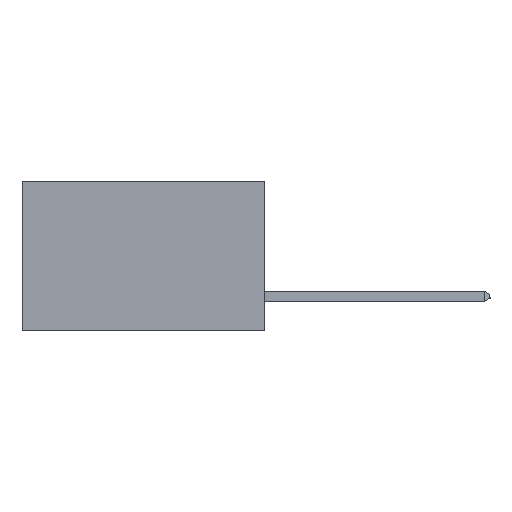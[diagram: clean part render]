
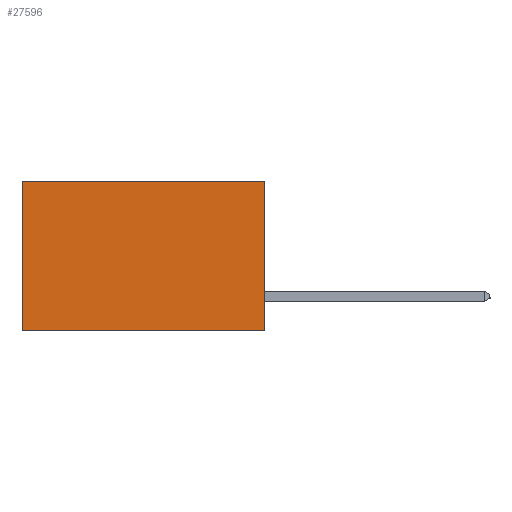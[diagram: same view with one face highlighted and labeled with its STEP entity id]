
A CAD part, left-side view. The second image highlights one B-rep face of the part: STEP entity #27596.
In plain terms, the highlighted planar face has unit normal (-1, 0, 0).
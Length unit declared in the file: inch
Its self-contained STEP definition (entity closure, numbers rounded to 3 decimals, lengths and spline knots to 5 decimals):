
#620 = ORIENTED_EDGE ( 'NONE', *, *, #14766, .F. ) ;
#2297 = VERTEX_POINT ( 'NONE', #15712 ) ;
#3064 = ORIENTED_EDGE ( 'NONE', *, *, #7268, .T. ) ;
#3065 = DIRECTION ( 'NONE',  ( 1., 0., 0. ) ) ;
#4919 = VECTOR ( 'NONE', #12209, 39.37008 ) ;
#7268 = EDGE_CURVE ( 'NONE', #17545, #28711, #10418, .T. ) ;
#8071 = CARTESIAN_POINT ( 'NONE',  ( 0.298, 0., 0. ) ) ;
#8106 = EDGE_CURVE ( 'NONE', #17545, #25234, #22474, .T. ) ;
#8983 = DIRECTION ( 'NONE',  ( 0., 0., -1. ) ) ;
#10080 = LINE ( 'NONE', #12280, #27967 ) ;
#10121 = EDGE_LOOP ( 'NONE', ( #15681, #620, #19511, #3064 ) ) ;
#10256 = CARTESIAN_POINT ( 'NONE',  ( 0.298, 0., 0. ) ) ;
#10418 = LINE ( 'NONE', #10256, #23617 ) ;
#10823 = AXIS2_PLACEMENT_3D ( 'NONE', #17030, #3065, #19365 ) ;
#12209 = DIRECTION ( 'NONE',  ( 0., 0., -1. ) ) ;
#12280 = CARTESIAN_POINT ( 'NONE',  ( 0.298, 0., -0.37 ) ) ;
#12533 = CARTESIAN_POINT ( 'NONE',  ( 0.298, 0., -0.37 ) ) ;
#12798 = FACE_OUTER_BOUND ( 'NONE', #10121, .T. ) ;
#14766 = EDGE_CURVE ( 'NONE', #25234, #2297, #10080, .T. ) ;
#15681 = ORIENTED_EDGE ( 'NONE', *, *, #25792, .T. ) ;
#15712 = CARTESIAN_POINT ( 'NONE',  ( 0.298, 0.6, -0.37 ) ) ;
#16213 = VECTOR ( 'NONE', #8983, 39.37008 ) ;
#17030 = CARTESIAN_POINT ( 'NONE',  ( 0.298, 0., 0. ) ) ;
#17310 = LINE ( 'NONE', #19145, #4919 ) ;
#17545 = VERTEX_POINT ( 'NONE', #8071 ) ;
#18893 = CARTESIAN_POINT ( 'NONE',  ( 0.298, 0.6, 0. ) ) ;
#19145 = CARTESIAN_POINT ( 'NONE',  ( 0.298, 0.6, 0. ) ) ;
#19365 = DIRECTION ( 'NONE',  ( 0., 0., -1. ) ) ;
#19511 = ORIENTED_EDGE ( 'NONE', *, *, #8106, .F. ) ;
#22474 = LINE ( 'NONE', #29871, #16213 ) ;
#23617 = VECTOR ( 'NONE', #26563, 39.37008 ) ;
#25234 = VERTEX_POINT ( 'NONE', #12533 ) ;
#25792 = EDGE_CURVE ( 'NONE', #28711, #2297, #17310, .T. ) ;
#26296 = DIRECTION ( 'NONE',  ( 0., 1., 0. ) ) ;
#26563 = DIRECTION ( 'NONE',  ( 0., 1., 0. ) ) ;
#27596 = ADVANCED_FACE ( 'NONE', ( #12798 ), #28678, .F. ) ;
#27967 = VECTOR ( 'NONE', #26296, 39.37008 ) ;
#28678 = PLANE ( 'NONE',  #10823 ) ;
#28711 = VERTEX_POINT ( 'NONE', #18893 ) ;
#29871 = CARTESIAN_POINT ( 'NONE',  ( 0.298, 0., 0. ) ) ;
